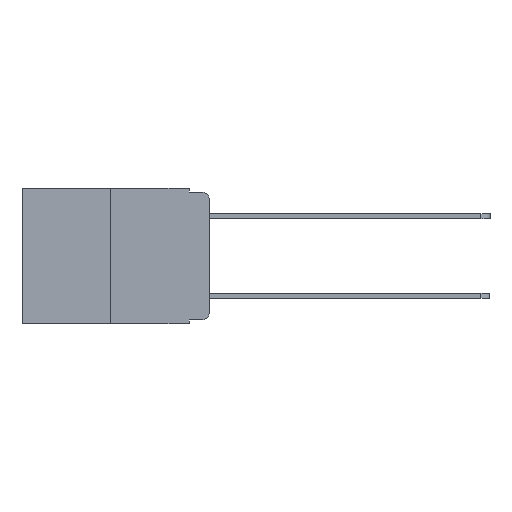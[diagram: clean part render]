
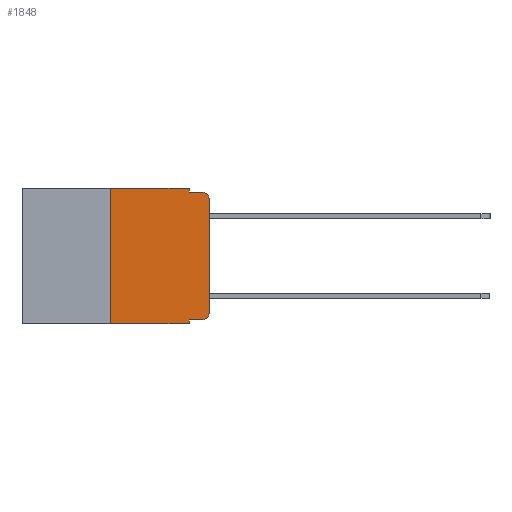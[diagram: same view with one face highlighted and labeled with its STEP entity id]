
A CAD part, left-side view. The second image highlights one B-rep face of the part: STEP entity #1848.
In plain terms, the highlighted planar face has unit normal (-1, 0, 0).
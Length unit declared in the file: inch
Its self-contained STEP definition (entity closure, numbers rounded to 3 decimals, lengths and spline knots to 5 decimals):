
#244 = EDGE_CURVE ( 'NONE', #1635, #6053, #5579, .T. ) ;
#512 = VERTEX_POINT ( 'NONE', #4720 ) ;
#621 = VERTEX_POINT ( 'NONE', #1394 ) ;
#1069 = CARTESIAN_POINT ( 'NONE',  ( 0., 0.051, -0.333 ) ) ;
#1394 = CARTESIAN_POINT ( 'NONE',  ( 0., 0., -0.313 ) ) ;
#1635 = VERTEX_POINT ( 'NONE', #6071 ) ;
#1738 = FACE_OUTER_BOUND ( 'NONE', #3724, .T. ) ;
#1741 = CIRCLE ( 'NONE', #8738, 0.02 ) ;
#1793 = ORIENTED_EDGE ( 'NONE', *, *, #4172, .T. ) ;
#1848 = ADVANCED_FACE ( 'NONE', ( #1738 ), #4627, .F. ) ;
#2246 = EDGE_CURVE ( 'NONE', #8550, #10279, #4830, .T. ) ;
#2351 = VECTOR ( 'NONE', #11541, 39.37008 ) ;
#2374 = DIRECTION ( 'NONE',  ( 0., 0., -1. ) ) ;
#2487 = LINE ( 'NONE', #5305, #12231 ) ;
#2711 = CARTESIAN_POINT ( 'NONE',  ( 0., 0.473, 0. ) ) ;
#2722 = VECTOR ( 'NONE', #3431, 39.37008 ) ;
#3031 = LINE ( 'NONE', #5424, #8437 ) ;
#3431 = DIRECTION ( 'NONE',  ( 0., -1., 0. ) ) ;
#3693 = CARTESIAN_POINT ( 'NONE',  ( 0., 0.473, 0. ) ) ;
#3715 = LINE ( 'NONE', #10715, #12384 ) ;
#3724 = EDGE_LOOP ( 'NONE', ( #1793, #5736, #8570, #6410, #8813, #7060, #4561, #7345, #11908, #10067 ) ) ;
#4172 = EDGE_CURVE ( 'NONE', #621, #5647, #2487, .T. ) ;
#4216 = EDGE_CURVE ( 'NONE', #5647, #10279, #1741, .T. ) ;
#4368 = DIRECTION ( 'NONE',  ( -1., 0., 0. ) ) ;
#4533 = DIRECTION ( 'NONE',  ( 1., 0., 0. ) ) ;
#4561 = ORIENTED_EDGE ( 'NONE', *, *, #5168, .T. ) ;
#4627 = PLANE ( 'NONE',  #6250 ) ;
#4720 = CARTESIAN_POINT ( 'NONE',  ( 0., 0.051, -0.333 ) ) ;
#4794 = CARTESIAN_POINT ( 'NONE',  ( 0., 0.473, -0.343 ) ) ;
#4805 = VERTEX_POINT ( 'NONE', #7989 ) ;
#4830 = LINE ( 'NONE', #8348, #7877 ) ;
#5168 = EDGE_CURVE ( 'NONE', #4805, #8971, #7453, .T. ) ;
#5305 = CARTESIAN_POINT ( 'NONE',  ( 0., 0., 0. ) ) ;
#5424 = CARTESIAN_POINT ( 'NONE',  ( 0., 0.051, 0. ) ) ;
#5579 = LINE ( 'NONE', #2711, #2722 ) ;
#5647 = VERTEX_POINT ( 'NONE', #8780 ) ;
#5736 = ORIENTED_EDGE ( 'NONE', *, *, #4216, .T. ) ;
#6053 = VERTEX_POINT ( 'NONE', #11593 ) ;
#6071 = CARTESIAN_POINT ( 'NONE',  ( 0., 0.25, 0. ) ) ;
#6250 = AXIS2_PLACEMENT_3D ( 'NONE', #3693, #4533, #2374 ) ;
#6410 = ORIENTED_EDGE ( 'NONE', *, *, #7116, .F. ) ;
#6575 = VECTOR ( 'NONE', #10903, 39.37008 ) ;
#6640 = CARTESIAN_POINT ( 'NONE',  ( 0., 0.02, -0.313 ) ) ;
#6796 = CARTESIAN_POINT ( 'NONE',  ( 0., 0.02, -0.01 ) ) ;
#7060 = ORIENTED_EDGE ( 'NONE', *, *, #7605, .F. ) ;
#7096 = CARTESIAN_POINT ( 'NONE',  ( 0., 0.02, -0.333 ) ) ;
#7116 = EDGE_CURVE ( 'NONE', #6053, #8550, #11041, .T. ) ;
#7345 = ORIENTED_EDGE ( 'NONE', *, *, #7606, .F. ) ;
#7453 = LINE ( 'NONE', #4794, #9405 ) ;
#7605 = EDGE_CURVE ( 'NONE', #4805, #1635, #3715, .T. ) ;
#7606 = EDGE_CURVE ( 'NONE', #512, #8971, #3031, .T. ) ;
#7621 = DIRECTION ( 'NONE',  ( 0., 0., -1. ) ) ;
#7624 = EDGE_CURVE ( 'NONE', #512, #11538, #8191, .T. ) ;
#7652 = EDGE_CURVE ( 'NONE', #11538, #621, #9806, .T. ) ;
#7877 = VECTOR ( 'NONE', #8314, 39.37008 ) ;
#7989 = CARTESIAN_POINT ( 'NONE',  ( 0., 0.25, -0.343 ) ) ;
#8191 = LINE ( 'NONE', #1069, #2351 ) ;
#8314 = DIRECTION ( 'NONE',  ( 0., -1., 0. ) ) ;
#8348 = CARTESIAN_POINT ( 'NONE',  ( 0., 0.051, -0.01 ) ) ;
#8372 = DIRECTION ( 'NONE',  ( 0., 0., -1. ) ) ;
#8437 = VECTOR ( 'NONE', #8372, 39.37008 ) ;
#8550 = VERTEX_POINT ( 'NONE', #10510 ) ;
#8570 = ORIENTED_EDGE ( 'NONE', *, *, #2246, .F. ) ;
#8738 = AXIS2_PLACEMENT_3D ( 'NONE', #9957, #4368, #10734 ) ;
#8780 = CARTESIAN_POINT ( 'NONE',  ( 0., 0., -0.03 ) ) ;
#8813 = ORIENTED_EDGE ( 'NONE', *, *, #244, .F. ) ;
#8971 = VERTEX_POINT ( 'NONE', #10017 ) ;
#9132 = DIRECTION ( 'NONE',  ( 0., 0., 1. ) ) ;
#9280 = CARTESIAN_POINT ( 'NONE',  ( 0., 0.051, 0. ) ) ;
#9405 = VECTOR ( 'NONE', #11836, 39.37008 ) ;
#9806 = CIRCLE ( 'NONE', #11208, 0.02 ) ;
#9957 = CARTESIAN_POINT ( 'NONE',  ( 0., 0.02, -0.03 ) ) ;
#10017 = CARTESIAN_POINT ( 'NONE',  ( 0., 0.051, -0.343 ) ) ;
#10067 = ORIENTED_EDGE ( 'NONE', *, *, #7652, .T. ) ;
#10279 = VERTEX_POINT ( 'NONE', #6796 ) ;
#10510 = CARTESIAN_POINT ( 'NONE',  ( 0., 0.051, -0.01 ) ) ;
#10715 = CARTESIAN_POINT ( 'NONE',  ( 0., 0.25, 0. ) ) ;
#10734 = DIRECTION ( 'NONE',  ( 0., 0., -1. ) ) ;
#10903 = DIRECTION ( 'NONE',  ( 0., 0., -1. ) ) ;
#11041 = LINE ( 'NONE', #9280, #6575 ) ;
#11208 = AXIS2_PLACEMENT_3D ( 'NONE', #6640, #12404, #7621 ) ;
#11538 = VERTEX_POINT ( 'NONE', #7096 ) ;
#11541 = DIRECTION ( 'NONE',  ( 0., -1., 0. ) ) ;
#11593 = CARTESIAN_POINT ( 'NONE',  ( 0., 0.051, 0. ) ) ;
#11836 = DIRECTION ( 'NONE',  ( 0., -1., 0. ) ) ;
#11908 = ORIENTED_EDGE ( 'NONE', *, *, #7624, .T. ) ;
#12221 = DIRECTION ( 'NONE',  ( 0., 0., 1. ) ) ;
#12231 = VECTOR ( 'NONE', #12221, 39.37008 ) ;
#12384 = VECTOR ( 'NONE', #9132, 39.37008 ) ;
#12404 = DIRECTION ( 'NONE',  ( -1., 0., 0. ) ) ;
